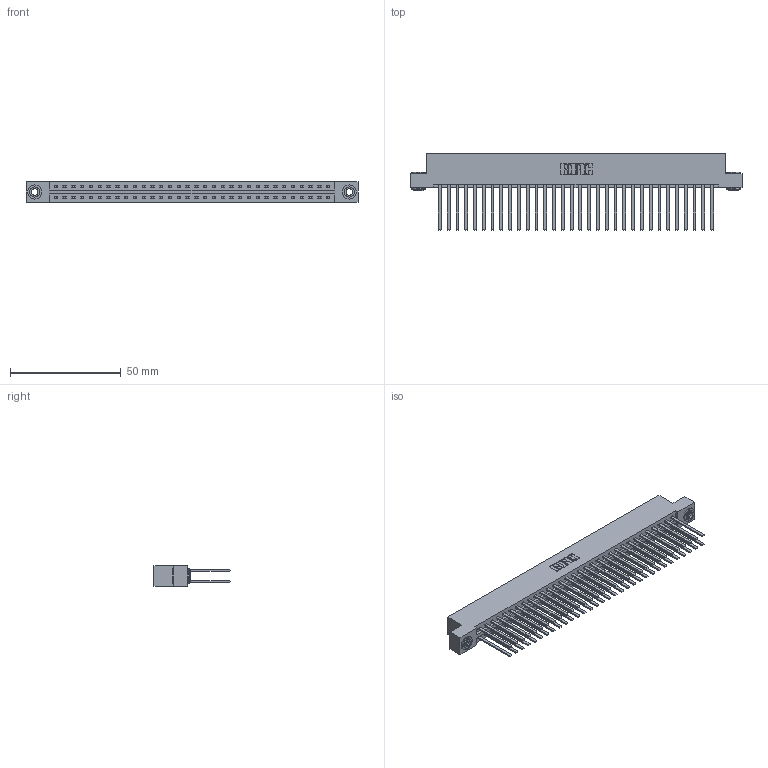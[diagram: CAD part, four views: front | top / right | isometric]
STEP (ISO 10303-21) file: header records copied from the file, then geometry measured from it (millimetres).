
FILE_DESCRIPTION (( 'STEP AP203' ), '1' );
FILE_NAME ('387-064-544-203.STEP', '2019-10-19T17:02:34', ( '' ), ( '' ), 'SwSTEP 2.0', 'SolidWorks 2016', '' );
FILE_SCHEMA (( 'CONFIG_CONTROL_DESIGN' ));
Length unit declared in the file: inch
Products named in the file (4): 387-064-544-203; 345-292-001_345-293-144; 345-250-002_345-250-002-102; 337 Part_Flush Mounting Lugs - 0.156 Dia-TH
Assembly tree (67 placements, depth 2):
  387-064-544-203
    337 Part_Flush Mounting Lugs - 0.156 Dia-TH
    345-292-001_345-293-144  x64
    345-250-002_345-250-002-102  x2
Bounding box: 149.81 x 34.3 x 9.4 mm (x, y, z)
Volume: 16571.5 mm3; surface area: 21792.2 mm2
Topology: 67 solids, 67 shells, 3224 faces, 9539 edges, 6270 vertices
Faces by surface type: plane 2256, cylinder 960, cone 8
Entity records: 26570 total; most frequent: CARTESIAN_POINT 4457, ORIENTED_EDGE 4386, DIRECTION 3839, EDGE_CURVE 2193, LINE 2045, VECTOR 2045, VERTEX_POINT 1458, AXIS2_PLACEMENT_3D 897
